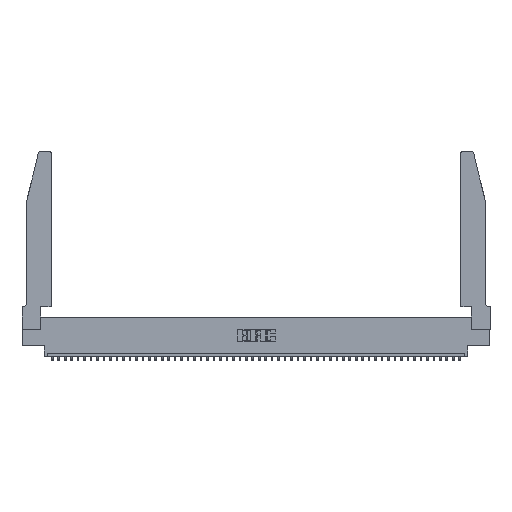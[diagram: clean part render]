
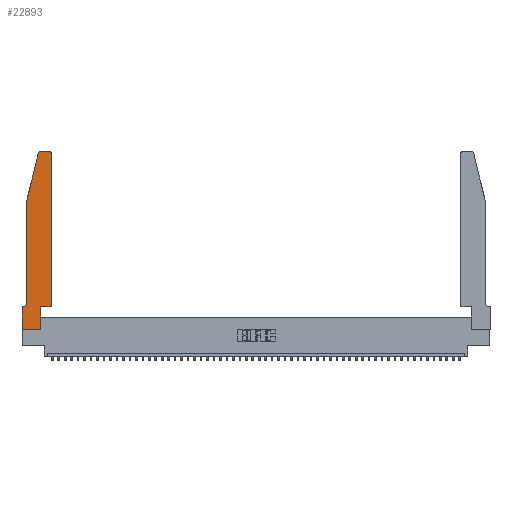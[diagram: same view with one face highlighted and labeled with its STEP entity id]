
A CAD part, top view. The second image highlights one B-rep face of the part: STEP entity #22893.
In plain terms, the highlighted planar face has unit normal (0, 0, 1).
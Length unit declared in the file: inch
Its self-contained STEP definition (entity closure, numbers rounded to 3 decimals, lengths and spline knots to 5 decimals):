
#476 = LINE ( 'NONE', #46003, #5951 ) ;
#1526 = CARTESIAN_POINT ( 'NONE',  ( 0., 0., 0.37 ) ) ;
#1624 = ORIENTED_EDGE ( 'NONE', *, *, #46982, .T. ) ;
#1880 = VERTEX_POINT ( 'NONE', #31700 ) ;
#2147 = CARTESIAN_POINT ( 'NONE',  ( 0.4205, 2.72, 0.37 ) ) ;
#2486 = DIRECTION ( 'NONE',  ( 0., 0., 1. ) ) ;
#2646 = CARTESIAN_POINT ( 'NONE',  ( 0.0755, 2., 0.37 ) ) ;
#3282 = LINE ( 'NONE', #43907, #17720 ) ;
#3285 = ORIENTED_EDGE ( 'NONE', *, *, #30562, .T. ) ;
#3975 = VECTOR ( 'NONE', #45611, 39.37008 ) ;
#4312 = EDGE_CURVE ( 'NONE', #25285, #13274, #35126, .T. ) ;
#5014 = CARTESIAN_POINT ( 'NONE',  ( 0., 0.35, 0.37 ) ) ;
#5033 = PLANE ( 'NONE',  #22967 ) ;
#5398 = DIRECTION ( 'NONE',  ( 1., 0., 0. ) ) ;
#5723 = EDGE_CURVE ( 'NONE', #23510, #45796, #476, .T. ) ;
#5951 = VECTOR ( 'NONE', #26131, 39.37008 ) ;
#6331 = AXIS2_PLACEMENT_3D ( 'NONE', #36102, #44303, #16981 ) ;
#8073 = EDGE_CURVE ( 'NONE', #1880, #23510, #36607, .T. ) ;
#8822 = DIRECTION ( 'NONE',  ( 0., 1., 0. ) ) ;
#9187 = EDGE_CURVE ( 'NONE', #43171, #38821, #15490, .T. ) ;
#9215 = VERTEX_POINT ( 'NONE', #2646 ) ;
#9244 = DIRECTION ( 'NONE',  ( 0., -1., 0. ) ) ;
#9288 = ORIENTED_EDGE ( 'NONE', *, *, #4312, .T. ) ;
#9775 = VERTEX_POINT ( 'NONE', #47724 ) ;
#9811 = CARTESIAN_POINT ( 'NONE',  ( 0.0755, 2., 0.37 ) ) ;
#9878 = LINE ( 'NONE', #16659, #25591 ) ;
#10380 = ORIENTED_EDGE ( 'NONE', *, *, #8073, .T. ) ;
#10986 = ORIENTED_EDGE ( 'NONE', *, *, #44358, .T. ) ;
#11149 = DIRECTION ( 'NONE',  ( -0.239, -0.971, 0. ) ) ;
#12973 = ORIENTED_EDGE ( 'NONE', *, *, #9187, .T. ) ;
#13274 = VERTEX_POINT ( 'NONE', #1526 ) ;
#14119 = CIRCLE ( 'NONE', #30131, 0.03 ) ;
#14650 = CARTESIAN_POINT ( 'NONE',  ( 0.4205, 2.75, 0.37 ) ) ;
#15388 = CARTESIAN_POINT ( 'NONE',  ( 0.2865, 0.35, 0.37 ) ) ;
#15490 = CIRCLE ( 'NONE', #28088, 0.03 ) ;
#15886 = LINE ( 'NONE', #33007, #41996 ) ;
#16315 = CARTESIAN_POINT ( 'NONE',  ( 0., 0.35, 0.37 ) ) ;
#16538 = LINE ( 'NONE', #40040, #20785 ) ;
#16659 = CARTESIAN_POINT ( 'NONE',  ( 0.0755, 2., 0.37 ) ) ;
#16981 = DIRECTION ( 'NONE',  ( -1., 0., 0. ) ) ;
#17296 = EDGE_CURVE ( 'NONE', #38821, #9215, #27285, .T. ) ;
#17680 = DIRECTION ( 'NONE',  ( 0., -1., 0. ) ) ;
#17720 = VECTOR ( 'NONE', #8822, 39.37008 ) ;
#20746 = CARTESIAN_POINT ( 'NONE',  ( 0.0055, 0.35, 0.37 ) ) ;
#20785 = VECTOR ( 'NONE', #43461, 39.37008 ) ;
#21119 = VERTEX_POINT ( 'NONE', #44277 ) ;
#21543 = CARTESIAN_POINT ( 'NONE',  ( 0.284, 2.72, 0.37 ) ) ;
#22659 = FACE_OUTER_BOUND ( 'NONE', #23552, .T. ) ;
#22668 = CARTESIAN_POINT ( 'NONE',  ( 0.2605, 2.75, 0.37 ) ) ;
#22735 = ORIENTED_EDGE ( 'NONE', *, *, #5723, .T. ) ;
#22893 = ADVANCED_FACE ( 'NONE', ( #22659 ), #5033, .T. ) ;
#22967 = AXIS2_PLACEMENT_3D ( 'NONE', #16315, #44162, #5398 ) ;
#23510 = VERTEX_POINT ( 'NONE', #46545 ) ;
#23552 = EDGE_LOOP ( 'NONE', ( #24560, #12973, #30370, #29204, #1624, #10986, #9288, #48336, #10380, #22735, #28164, #3285 ) ) ;
#24069 = EDGE_CURVE ( 'NONE', #45796, #9775, #3282, .T. ) ;
#24560 = ORIENTED_EDGE ( 'NONE', *, *, #36738, .T. ) ;
#25049 = VERTEX_POINT ( 'NONE', #14650 ) ;
#25285 = VERTEX_POINT ( 'NONE', #5014 ) ;
#25591 = VECTOR ( 'NONE', #9244, 39.37008 ) ;
#26131 = DIRECTION ( 'NONE',  ( 1., 0., 0. ) ) ;
#26571 = VERTEX_POINT ( 'NONE', #20746 ) ;
#27285 = LINE ( 'NONE', #9811, #29086 ) ;
#27868 = VECTOR ( 'NONE', #17680, 39.37008 ) ;
#28088 = AXIS2_PLACEMENT_3D ( 'NONE', #21543, #44937, #49197 ) ;
#28164 = ORIENTED_EDGE ( 'NONE', *, *, #24069, .T. ) ;
#28239 = CARTESIAN_POINT ( 'NONE',  ( 0.4505, 0.35, 0.37 ) ) ;
#28734 = LINE ( 'NONE', #22668, #3975 ) ;
#29086 = VECTOR ( 'NONE', #11149, 39.37008 ) ;
#29204 = ORIENTED_EDGE ( 'NONE', *, *, #44424, .T. ) ;
#30131 = AXIS2_PLACEMENT_3D ( 'NONE', #2147, #2486, #37428 ) ;
#30370 = ORIENTED_EDGE ( 'NONE', *, *, #17296, .T. ) ;
#30562 = EDGE_CURVE ( 'NONE', #9775, #25049, #14119, .T. ) ;
#30630 = DIRECTION ( 'NONE',  ( 0., 1., 0. ) ) ;
#31700 = CARTESIAN_POINT ( 'NONE',  ( 0.2865, 0., 0.37 ) ) ;
#32384 = VECTOR ( 'NONE', #30630, 39.37008 ) ;
#33007 = CARTESIAN_POINT ( 'NONE',  ( 0., 0., 0.37 ) ) ;
#35126 = LINE ( 'NONE', #48913, #27868 ) ;
#36102 = CARTESIAN_POINT ( 'NONE',  ( 0.0055, 0.42, 0.37 ) ) ;
#36136 = CIRCLE ( 'NONE', #6331, 0.07 ) ;
#36607 = LINE ( 'NONE', #15388, #32384 ) ;
#36738 = EDGE_CURVE ( 'NONE', #25049, #43171, #28734, .T. ) ;
#37428 = DIRECTION ( 'NONE',  ( 1., 0., 0. ) ) ;
#38821 = VERTEX_POINT ( 'NONE', #46628 ) ;
#40040 = CARTESIAN_POINT ( 'NONE',  ( 0.0755, 0.35, 0.37 ) ) ;
#41996 = VECTOR ( 'NONE', #48130, 39.37008 ) ;
#43171 = VERTEX_POINT ( 'NONE', #47340 ) ;
#43461 = DIRECTION ( 'NONE',  ( -1., 0., 0. ) ) ;
#43831 = EDGE_CURVE ( 'NONE', #13274, #1880, #15886, .T. ) ;
#43907 = CARTESIAN_POINT ( 'NONE',  ( 0.4505, 0.35, 0.37 ) ) ;
#44162 = DIRECTION ( 'NONE',  ( 0., 0., 1. ) ) ;
#44277 = CARTESIAN_POINT ( 'NONE',  ( 0.0755, 0.42, 0.37 ) ) ;
#44303 = DIRECTION ( 'NONE',  ( 0., 0., -1. ) ) ;
#44358 = EDGE_CURVE ( 'NONE', #26571, #25285, #16538, .T. ) ;
#44424 = EDGE_CURVE ( 'NONE', #9215, #21119, #9878, .T. ) ;
#44937 = DIRECTION ( 'NONE',  ( 0., 0., 1. ) ) ;
#45611 = DIRECTION ( 'NONE',  ( -1., 0., 0. ) ) ;
#45796 = VERTEX_POINT ( 'NONE', #28239 ) ;
#46003 = CARTESIAN_POINT ( 'NONE',  ( 0.4505, 0.35, 0.37 ) ) ;
#46545 = CARTESIAN_POINT ( 'NONE',  ( 0.2865, 0.35, 0.37 ) ) ;
#46628 = CARTESIAN_POINT ( 'NONE',  ( 0.25487, 2.72718, 0.37 ) ) ;
#46982 = EDGE_CURVE ( 'NONE', #21119, #26571, #36136, .T. ) ;
#47340 = CARTESIAN_POINT ( 'NONE',  ( 0.284, 2.75, 0.37 ) ) ;
#47724 = CARTESIAN_POINT ( 'NONE',  ( 0.4505, 2.72, 0.37 ) ) ;
#48130 = DIRECTION ( 'NONE',  ( 1., 0., 0. ) ) ;
#48336 = ORIENTED_EDGE ( 'NONE', *, *, #43831, .T. ) ;
#48913 = CARTESIAN_POINT ( 'NONE',  ( 0., 0., 0.37 ) ) ;
#49197 = DIRECTION ( 'NONE',  ( 1., 0., 0. ) ) ;
